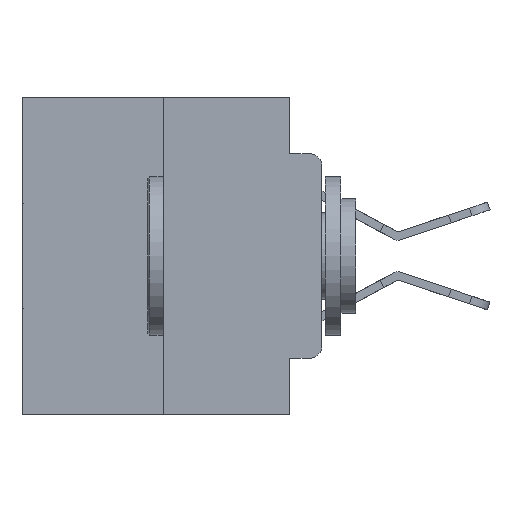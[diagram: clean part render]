
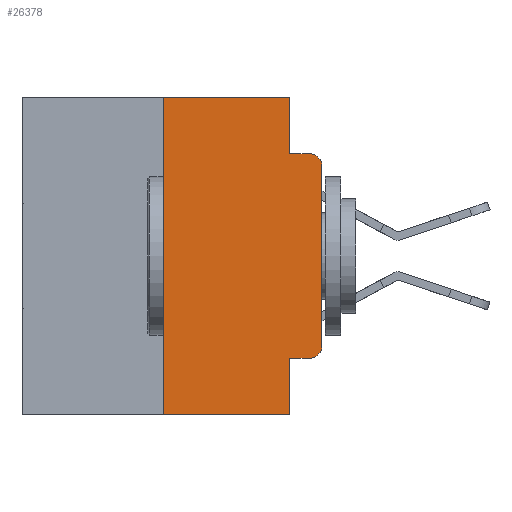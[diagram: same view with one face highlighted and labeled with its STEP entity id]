
A CAD part, left-side view. The second image highlights one B-rep face of the part: STEP entity #26378.
In plain terms, the highlighted planar face has unit normal (-1, 0, 0).
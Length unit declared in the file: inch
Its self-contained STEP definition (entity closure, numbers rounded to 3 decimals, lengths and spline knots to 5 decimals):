
#218 = AXIS2_PLACEMENT_3D ( 'NONE', #9980, #7183, #5032 ) ;
#551 = VERTEX_POINT ( 'NONE', #6711 ) ;
#586 = VERTEX_POINT ( 'NONE', #28475 ) ;
#880 = LINE ( 'NONE', #1693, #25187 ) ;
#1094 = CARTESIAN_POINT ( 'NONE',  ( 0., 0.25, 0. ) ) ;
#1392 = VECTOR ( 'NONE', #29177, 39.37008 ) ;
#1693 = CARTESIAN_POINT ( 'NONE',  ( 0., 0.051, -0.0885 ) ) ;
#1773 = ORIENTED_EDGE ( 'NONE', *, *, #4731, .T. ) ;
#2421 = PLANE ( 'NONE',  #19477 ) ;
#3920 = CARTESIAN_POINT ( 'NONE',  ( 0., 0.25, 0. ) ) ;
#4731 = EDGE_CURVE ( 'NONE', #5884, #26077, #20043, .T. ) ;
#4871 = CARTESIAN_POINT ( 'NONE',  ( 0., 0.02, -0.4115 ) ) ;
#5032 = DIRECTION ( 'NONE',  ( 0., 0., -1. ) ) ;
#5452 = ORIENTED_EDGE ( 'NONE', *, *, #29225, .F. ) ;
#5465 = EDGE_CURVE ( 'NONE', #551, #21270, #18558, .T. ) ;
#5884 = VERTEX_POINT ( 'NONE', #11801 ) ;
#6711 = CARTESIAN_POINT ( 'NONE',  ( 0., 0.051, 0. ) ) ;
#6857 = LINE ( 'NONE', #22792, #20528 ) ;
#7183 = DIRECTION ( 'NONE',  ( -1., 0., 0. ) ) ;
#7433 = DIRECTION ( 'NONE',  ( -1., 0., 0. ) ) ;
#7622 = DIRECTION ( 'NONE',  ( 0., 0., -1. ) ) ;
#7809 = EDGE_CURVE ( 'NONE', #26077, #17456, #15888, .T. ) ;
#8165 = FACE_OUTER_BOUND ( 'NONE', #13824, .T. ) ;
#9210 = DIRECTION ( 'NONE',  ( 0., 0., -1. ) ) ;
#9948 = VECTOR ( 'NONE', #20133, 39.37008 ) ;
#9980 = CARTESIAN_POINT ( 'NONE',  ( 0., 0.02, -0.1085 ) ) ;
#10486 = CARTESIAN_POINT ( 'NONE',  ( 0., 0., -0.1085 ) ) ;
#10888 = CARTESIAN_POINT ( 'NONE',  ( 0., 0.051, 0. ) ) ;
#10968 = CARTESIAN_POINT ( 'NONE',  ( 0., 0.051, -0.4115 ) ) ;
#11484 = EDGE_CURVE ( 'NONE', #586, #21363, #16250, .T. ) ;
#11515 = CARTESIAN_POINT ( 'NONE',  ( 0., 0.473, 0. ) ) ;
#11801 = CARTESIAN_POINT ( 'NONE',  ( 0., 0., -0.3915 ) ) ;
#13026 = CARTESIAN_POINT ( 'NONE',  ( 0., 0.051, -0.5 ) ) ;
#13165 = DIRECTION ( 'NONE',  ( 0., 0., -1. ) ) ;
#13696 = ORIENTED_EDGE ( 'NONE', *, *, #14066, .F. ) ;
#13824 = EDGE_LOOP ( 'NONE', ( #1773, #18916, #18316, #17592, #14624, #13696, #29167, #5452, #27613, #16271 ) ) ;
#13887 = DIRECTION ( 'NONE',  ( 1., 0., 0. ) ) ;
#14066 = EDGE_CURVE ( 'NONE', #29903, #28988, #17531, .T. ) ;
#14624 = ORIENTED_EDGE ( 'NONE', *, *, #19942, .F. ) ;
#14904 = CARTESIAN_POINT ( 'NONE',  ( 0., 0.473, -0.5 ) ) ;
#15342 = EDGE_CURVE ( 'NONE', #21270, #17456, #880, .T. ) ;
#15849 = DIRECTION ( 'NONE',  ( 0., -1., 0. ) ) ;
#15888 = CIRCLE ( 'NONE', #218, 0.02 ) ;
#16107 = DIRECTION ( 'NONE',  ( 0., -1., 0. ) ) ;
#16250 = LINE ( 'NONE', #10968, #9948 ) ;
#16271 = ORIENTED_EDGE ( 'NONE', *, *, #18595, .T. ) ;
#16516 = LINE ( 'NONE', #14904, #1392 ) ;
#17214 = CIRCLE ( 'NONE', #26407, 0.02 ) ;
#17278 = VECTOR ( 'NONE', #25893, 39.37008 ) ;
#17456 = VERTEX_POINT ( 'NONE', #17930 ) ;
#17531 = LINE ( 'NONE', #3920, #17879 ) ;
#17592 = ORIENTED_EDGE ( 'NONE', *, *, #5465, .F. ) ;
#17879 = VECTOR ( 'NONE', #20194, 39.37008 ) ;
#17930 = CARTESIAN_POINT ( 'NONE',  ( 0., 0.02, -0.0885 ) ) ;
#18313 = CARTESIAN_POINT ( 'NONE',  ( 0., 0.051, -0.0885 ) ) ;
#18316 = ORIENTED_EDGE ( 'NONE', *, *, #15342, .F. ) ;
#18558 = LINE ( 'NONE', #10888, #27362 ) ;
#18595 = EDGE_CURVE ( 'NONE', #21363, #5884, #17214, .T. ) ;
#18916 = ORIENTED_EDGE ( 'NONE', *, *, #7809, .T. ) ;
#19070 = CARTESIAN_POINT ( 'NONE',  ( 0., 0.25, -0.5 ) ) ;
#19477 = AXIS2_PLACEMENT_3D ( 'NONE', #11515, #13887, #9210 ) ;
#19731 = EDGE_CURVE ( 'NONE', #29903, #29700, #16516, .T. ) ;
#19942 = EDGE_CURVE ( 'NONE', #28988, #551, #6857, .T. ) ;
#20043 = LINE ( 'NONE', #23897, #28186 ) ;
#20133 = DIRECTION ( 'NONE',  ( 0., -1., 0. ) ) ;
#20194 = DIRECTION ( 'NONE',  ( 0., 0., 1. ) ) ;
#20528 = VECTOR ( 'NONE', #16107, 39.37008 ) ;
#21239 = DIRECTION ( 'NONE',  ( 0., 0., 1. ) ) ;
#21270 = VERTEX_POINT ( 'NONE', #18313 ) ;
#21363 = VERTEX_POINT ( 'NONE', #4871 ) ;
#22792 = CARTESIAN_POINT ( 'NONE',  ( 0., 0.473, 0. ) ) ;
#23426 = CARTESIAN_POINT ( 'NONE',  ( 0., 0.051, 0. ) ) ;
#23897 = CARTESIAN_POINT ( 'NONE',  ( 0., 0., 0. ) ) ;
#25187 = VECTOR ( 'NONE', #15849, 39.37008 ) ;
#25893 = DIRECTION ( 'NONE',  ( 0., 0., -1. ) ) ;
#26077 = VERTEX_POINT ( 'NONE', #10486 ) ;
#26378 = ADVANCED_FACE ( 'NONE', ( #8165 ), #2421, .F. ) ;
#26407 = AXIS2_PLACEMENT_3D ( 'NONE', #28891, #7433, #7622 ) ;
#27362 = VECTOR ( 'NONE', #13165, 39.37008 ) ;
#27613 = ORIENTED_EDGE ( 'NONE', *, *, #11484, .T. ) ;
#28186 = VECTOR ( 'NONE', #21239, 39.37008 ) ;
#28475 = CARTESIAN_POINT ( 'NONE',  ( 0., 0.051, -0.4115 ) ) ;
#28891 = CARTESIAN_POINT ( 'NONE',  ( 0., 0.02, -0.3915 ) ) ;
#28988 = VERTEX_POINT ( 'NONE', #1094 ) ;
#29167 = ORIENTED_EDGE ( 'NONE', *, *, #19731, .T. ) ;
#29177 = DIRECTION ( 'NONE',  ( 0., -1., 0. ) ) ;
#29225 = EDGE_CURVE ( 'NONE', #586, #29700, #29782, .T. ) ;
#29700 = VERTEX_POINT ( 'NONE', #13026 ) ;
#29782 = LINE ( 'NONE', #23426, #17278 ) ;
#29903 = VERTEX_POINT ( 'NONE', #19070 ) ;
